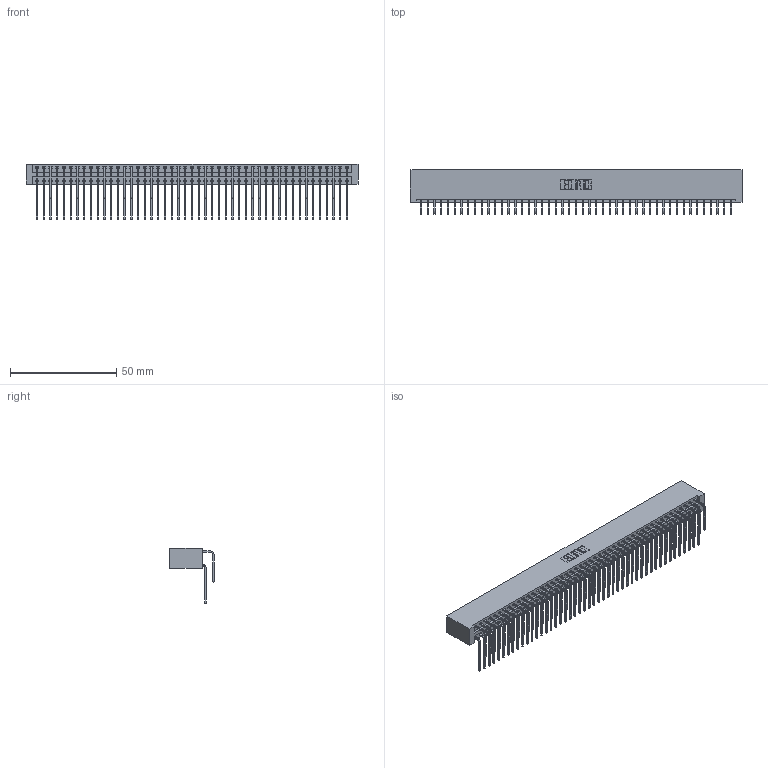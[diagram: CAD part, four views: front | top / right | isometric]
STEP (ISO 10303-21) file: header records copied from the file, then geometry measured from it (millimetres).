
FILE_DESCRIPTION (( 'STEP AP203' ), '1' );
FILE_NAME ('346-094-559-201.STEP', '2018-08-30T05:56:41', ( '' ), ( '' ), 'SwSTEP 2.0', 'SolidWorks 2016', '' );
FILE_SCHEMA (( 'CONFIG_CONTROL_DESIGN' ));
Length unit declared in the file: inch
Products named in the file (4): 346-094-559-201; 346 Part_No Mounting Lugs; 345-292-001_558 559 Tail - 1; 345-292-001_559 Tail - 2
Assembly tree (95 placements, depth 2):
  346-094-559-201
    346 Part_No Mounting Lugs
    345-292-001_558 559 Tail - 1  x47
    345-292-001_559 Tail - 2  x47
Bounding box: 156.46 x 20.89 x 26.16 mm (x, y, z)
Volume: 16411.6 mm3; surface area: 25402 mm2
Topology: 95 solids, 95 shells, 5190 faces, 15439 edges, 10166 vertices
Faces by surface type: plane 3550, cylinder 1640
Entity records: 31507 total; most frequent: CARTESIAN_POINT 5235, ORIENTED_EDGE 5118, DIRECTION 4631, EDGE_CURVE 2559, VECTOR 2207, LINE 2207, VERTEX_POINT 1702, AXIS2_PLACEMENT_3D 1212
